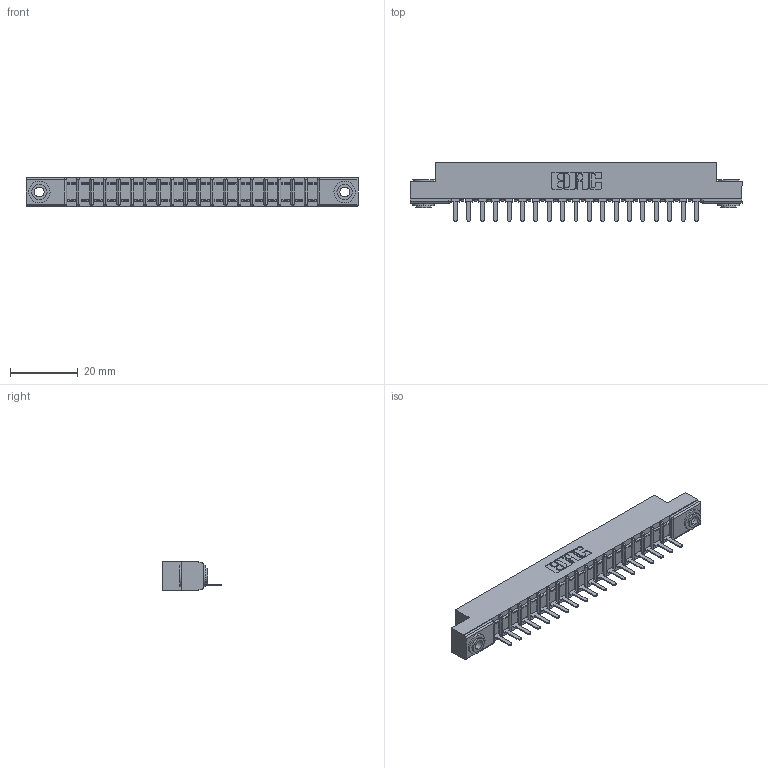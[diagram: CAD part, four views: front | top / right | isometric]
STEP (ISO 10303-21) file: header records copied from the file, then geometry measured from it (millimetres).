
FILE_DESCRIPTION (( 'STEP AP203' ), '1' );
FILE_NAME ('357-019-521-103.STEP', '2019-09-16T21:49:37', ( '' ), ( '' ), 'SwSTEP 2.0', 'SolidWorks 2016', '' );
FILE_SCHEMA (( 'CONFIG_CONTROL_DESIGN' ));
Length unit declared in the file: inch
Products named in the file (4): 357-019-521-103; 345-250-002_345-250-002-102; 307 Part_.156 Dia Mounting Holes; 307-290-002_521
Assembly tree (22 placements, depth 2):
  357-019-521-103
    307 Part_.156 Dia Mounting Holes
    307-290-002_521  x19
    345-250-002_345-250-002-102  x2
Bounding box: 98.3 x 17.42 x 8.71 mm (x, y, z)
Volume: 6490.3 mm3; surface area: 11893.3 mm2
Topology: 22 solids, 22 shells, 1596 faces, 4843 edges, 3170 vertices
Faces by surface type: plane 949, cylinder 599, sphere 40, cone 8
Entity records: 20907 total; most frequent: CARTESIAN_POINT 3501, ORIENTED_EDGE 3482, DIRECTION 3427, EDGE_CURVE 1741, VECTOR 1315, LINE 1315, VERTEX_POINT 1130, AXIS2_PLACEMENT_3D 1056
